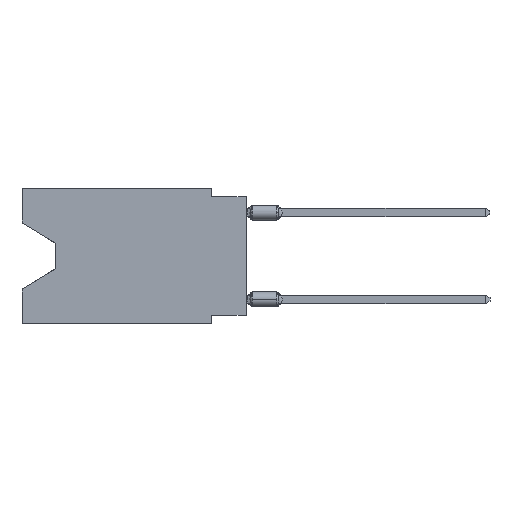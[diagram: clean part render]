
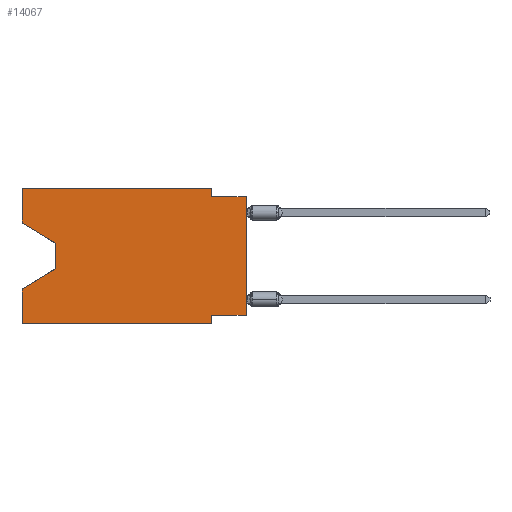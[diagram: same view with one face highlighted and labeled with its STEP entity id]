
A CAD part, left-side view. The second image highlights one B-rep face of the part: STEP entity #14067.
In plain terms, the highlighted planar face has unit normal (-1, 0, 0).
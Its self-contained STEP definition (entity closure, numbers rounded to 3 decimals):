
#47 = DIRECTION ( 'NONE',  ( 0., 0., -1. ) ) ;
#159 = ORIENTED_EDGE ( 'NONE', *, *, #1171, .F. ) ;
#1047 = CARTESIAN_POINT ( 'NONE',  ( 0., 2.54, -9.906 ) ) ;
#1171 = EDGE_CURVE ( 'NONE', #19546, #17290, #15871, .T. ) ;
#1254 = DIRECTION ( 'NONE',  ( 1., 0., 0. ) ) ;
#1494 = DIRECTION ( 'NONE',  ( 0., 0., 1. ) ) ;
#1839 = VECTOR ( 'NONE', #5728, 1000. ) ;
#2161 = VERTEX_POINT ( 'NONE', #3183 ) ;
#2178 = CARTESIAN_POINT ( 'NONE',  ( 0., 16.383, 0. ) ) ;
#2244 = ORIENTED_EDGE ( 'NONE', *, *, #23504, .F. ) ;
#2491 = ORIENTED_EDGE ( 'NONE', *, *, #11250, .F. ) ;
#2643 = ORIENTED_EDGE ( 'NONE', *, *, #20674, .F. ) ;
#3183 = CARTESIAN_POINT ( 'NONE',  ( 0., 2.54, 0. ) ) ;
#3210 = CARTESIAN_POINT ( 'NONE',  ( 0., 0., -0.635 ) ) ;
#3281 = VERTEX_POINT ( 'NONE', #19707 ) ;
#3300 = EDGE_CURVE ( 'NONE', #8063, #5221, #15908, .T. ) ;
#3335 = PLANE ( 'NONE',  #18560 ) ;
#3371 = CARTESIAN_POINT ( 'NONE',  ( 0., 2.54, -9.906 ) ) ;
#3610 = VECTOR ( 'NONE', #21630, 1000. ) ;
#3719 = VERTEX_POINT ( 'NONE', #4999 ) ;
#4007 = DIRECTION ( 'NONE',  ( 0., -1., 0. ) ) ;
#4135 = EDGE_CURVE ( 'NONE', #7417, #9386, #21964, .T. ) ;
#4680 = CARTESIAN_POINT ( 'NONE',  ( 0., 16.383, -9.906 ) ) ;
#4914 = LINE ( 'NONE', #14326, #7869 ) ;
#4999 = CARTESIAN_POINT ( 'NONE',  ( 0., 2.54, -0.635 ) ) ;
#5221 = VERTEX_POINT ( 'NONE', #5709 ) ;
#5243 = LINE ( 'NONE', #23719, #3610 ) ;
#5530 = DIRECTION ( 'NONE',  ( 0., 0., -1. ) ) ;
#5631 = VECTOR ( 'NONE', #1494, 1000. ) ;
#5661 = DIRECTION ( 'NONE',  ( 0., -1., 0. ) ) ;
#5709 = CARTESIAN_POINT ( 'NONE',  ( 0., 16.383, -7.36 ) ) ;
#5728 = DIRECTION ( 'NONE',  ( 0., 0., 1. ) ) ;
#6116 = CARTESIAN_POINT ( 'NONE',  ( 0., 13.97, -4.013 ) ) ;
#6595 = CARTESIAN_POINT ( 'NONE',  ( 0., 0., -9.271 ) ) ;
#7417 = VERTEX_POINT ( 'NONE', #16534 ) ;
#7424 = LINE ( 'NONE', #11202, #23647 ) ;
#7869 = VECTOR ( 'NONE', #11995, 1000. ) ;
#7876 = VERTEX_POINT ( 'NONE', #6116 ) ;
#7892 = VECTOR ( 'NONE', #5661, 1000. ) ;
#8063 = VERTEX_POINT ( 'NONE', #12645 ) ;
#8410 = VECTOR ( 'NONE', #17572, 1000. ) ;
#9026 = VECTOR ( 'NONE', #12115, 1000. ) ;
#9386 = VERTEX_POINT ( 'NONE', #1047 ) ;
#10572 = DIRECTION ( 'NONE',  ( 0., 0., -1. ) ) ;
#10606 = VERTEX_POINT ( 'NONE', #10847 ) ;
#10847 = CARTESIAN_POINT ( 'NONE',  ( 0., 0., -9.271 ) ) ;
#11019 = CARTESIAN_POINT ( 'NONE',  ( 0., 16.383, 0. ) ) ;
#11138 = CARTESIAN_POINT ( 'NONE',  ( 0., 0., 0. ) ) ;
#11202 = CARTESIAN_POINT ( 'NONE',  ( 0., 0., -0.635 ) ) ;
#11250 = EDGE_CURVE ( 'NONE', #2161, #3719, #4914, .T. ) ;
#11354 = EDGE_CURVE ( 'NONE', #3281, #9386, #21421, .T. ) ;
#11692 = CARTESIAN_POINT ( 'NONE',  ( 0., 16.383, -2.546 ) ) ;
#11995 = DIRECTION ( 'NONE',  ( 0., 0., -1. ) ) ;
#12115 = DIRECTION ( 'NONE',  ( 0., -1., 0. ) ) ;
#12245 = ORIENTED_EDGE ( 'NONE', *, *, #16007, .F. ) ;
#12550 = VECTOR ( 'NONE', #10572, 1000. ) ;
#12579 = VECTOR ( 'NONE', #19328, 1000. ) ;
#12609 = LINE ( 'NONE', #11138, #5631 ) ;
#12645 = CARTESIAN_POINT ( 'NONE',  ( 0., 13.97, -5.893 ) ) ;
#12784 = VERTEX_POINT ( 'NONE', #3210 ) ;
#13669 = ORIENTED_EDGE ( 'NONE', *, *, #11354, .T. ) ;
#13721 = ORIENTED_EDGE ( 'NONE', *, *, #16070, .T. ) ;
#14067 = ADVANCED_FACE ( 'NONE', ( #24125 ), #3335, .F. ) ;
#14184 = ORIENTED_EDGE ( 'NONE', *, *, #18984, .T. ) ;
#14326 = CARTESIAN_POINT ( 'NONE',  ( 0., 2.54, 0. ) ) ;
#14957 = CARTESIAN_POINT ( 'NONE',  ( 0., 16.383, 0. ) ) ;
#15344 = CARTESIAN_POINT ( 'NONE',  ( 0., 13.97, -5.893 ) ) ;
#15496 = EDGE_CURVE ( 'NONE', #17290, #2161, #22904, .T. ) ;
#15698 = ORIENTED_EDGE ( 'NONE', *, *, #21064, .T. ) ;
#15722 = CARTESIAN_POINT ( 'NONE',  ( 0., 16.383, 0. ) ) ;
#15871 = LINE ( 'NONE', #23341, #8410 ) ;
#15908 = LINE ( 'NONE', #15344, #16433 ) ;
#16007 = EDGE_CURVE ( 'NONE', #10606, #7417, #21151, .T. ) ;
#16070 = EDGE_CURVE ( 'NONE', #19546, #7876, #5243, .T. ) ;
#16433 = VECTOR ( 'NONE', #23254, 1000. ) ;
#16534 = CARTESIAN_POINT ( 'NONE',  ( 0., 2.54, -9.271 ) ) ;
#16682 = LINE ( 'NONE', #24157, #20921 ) ;
#16909 = ORIENTED_EDGE ( 'NONE', *, *, #15496, .F. ) ;
#17085 = LINE ( 'NONE', #2178, #1839 ) ;
#17290 = VERTEX_POINT ( 'NONE', #15722 ) ;
#17572 = DIRECTION ( 'NONE',  ( 0., 0., 1. ) ) ;
#18560 = AXIS2_PLACEMENT_3D ( 'NONE', #11019, #1254, #5530 ) ;
#18984 = EDGE_CURVE ( 'NONE', #10606, #12784, #12609, .T. ) ;
#19328 = DIRECTION ( 'NONE',  ( 0., 1., 0. ) ) ;
#19546 = VERTEX_POINT ( 'NONE', #11692 ) ;
#19707 = CARTESIAN_POINT ( 'NONE',  ( 0., 16.383, -9.906 ) ) ;
#19871 = EDGE_LOOP ( 'NONE', ( #13721, #15698, #20572, #2244, #13669, #22090, #12245, #14184, #2643, #2491, #16909, #159 ) ) ;
#20572 = ORIENTED_EDGE ( 'NONE', *, *, #3300, .T. ) ;
#20674 = EDGE_CURVE ( 'NONE', #3719, #12784, #7424, .T. ) ;
#20921 = VECTOR ( 'NONE', #47, 1000. ) ;
#21064 = EDGE_CURVE ( 'NONE', #7876, #8063, #16682, .T. ) ;
#21151 = LINE ( 'NONE', #6595, #12579 ) ;
#21421 = LINE ( 'NONE', #4680, #9026 ) ;
#21630 = DIRECTION ( 'NONE',  ( 0., -0.855, -0.519 ) ) ;
#21964 = LINE ( 'NONE', #3371, #12550 ) ;
#22090 = ORIENTED_EDGE ( 'NONE', *, *, #4135, .F. ) ;
#22904 = LINE ( 'NONE', #14957, #7892 ) ;
#23254 = DIRECTION ( 'NONE',  ( 0., 0.855, -0.519 ) ) ;
#23341 = CARTESIAN_POINT ( 'NONE',  ( 0., 16.383, 0. ) ) ;
#23504 = EDGE_CURVE ( 'NONE', #3281, #5221, #17085, .T. ) ;
#23647 = VECTOR ( 'NONE', #4007, 1000. ) ;
#23719 = CARTESIAN_POINT ( 'NONE',  ( 0., 16.383, -2.546 ) ) ;
#24125 = FACE_OUTER_BOUND ( 'NONE', #19871, .T. ) ;
#24157 = CARTESIAN_POINT ( 'NONE',  ( 0., 13.97, -4.013 ) ) ;
